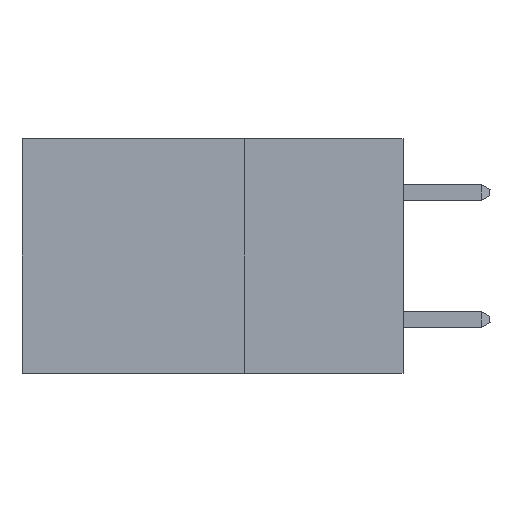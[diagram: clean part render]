
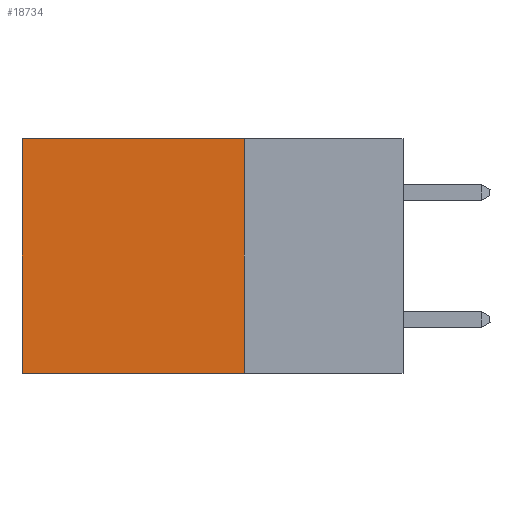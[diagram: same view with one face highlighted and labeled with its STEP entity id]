
A CAD part, left-side view. The second image highlights one B-rep face of the part: STEP entity #18734.
In plain terms, the highlighted planar face has unit normal (-1, 0, 0).
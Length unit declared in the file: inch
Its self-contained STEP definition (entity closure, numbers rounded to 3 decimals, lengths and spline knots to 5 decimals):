
#286 = LINE ( 'NONE', #6013, #18347 ) ;
#1853 = DIRECTION ( 'NONE',  ( 0., 1., 0. ) ) ;
#3866 = ORIENTED_EDGE ( 'NONE', *, *, #15349, .F. ) ;
#4247 = CARTESIAN_POINT ( 'NONE',  ( 0.2875, 0.6, 0. ) ) ;
#4672 = PLANE ( 'NONE',  #9237 ) ;
#4732 = DIRECTION ( 'NONE',  ( 0., 0., -1. ) ) ;
#5670 = LINE ( 'NONE', #18935, #10501 ) ;
#6013 = CARTESIAN_POINT ( 'NONE',  ( 0.2875, 0.25, 0. ) ) ;
#6296 = VERTEX_POINT ( 'NONE', #9944 ) ;
#7270 = ORIENTED_EDGE ( 'NONE', *, *, #11937, .F. ) ;
#7334 = EDGE_CURVE ( 'NONE', #19395, #7934, #16659, .T. ) ;
#7934 = VERTEX_POINT ( 'NONE', #17680 ) ;
#8270 = CARTESIAN_POINT ( 'NONE',  ( 0.2875, 0.25, 0. ) ) ;
#9197 = VECTOR ( 'NONE', #18101, 39.37008 ) ;
#9237 = AXIS2_PLACEMENT_3D ( 'NONE', #18799, #9454, #4732 ) ;
#9454 = DIRECTION ( 'NONE',  ( 1., 0., 0. ) ) ;
#9944 = CARTESIAN_POINT ( 'NONE',  ( 0.2875, 0.25, -0.37 ) ) ;
#9947 = DIRECTION ( 'NONE',  ( 0., 1., 0. ) ) ;
#9979 = VERTEX_POINT ( 'NONE', #16323 ) ;
#10481 = LINE ( 'NONE', #8270, #17430 ) ;
#10501 = VECTOR ( 'NONE', #1853, 39.37008 ) ;
#10537 = DIRECTION ( 'NONE',  ( 0., 0., -1. ) ) ;
#11758 = FACE_OUTER_BOUND ( 'NONE', #12238, .T. ) ;
#11937 = EDGE_CURVE ( 'NONE', #6296, #7934, #5670, .T. ) ;
#12238 = EDGE_LOOP ( 'NONE', ( #15682, #7270, #3866, #17017 ) ) ;
#12253 = EDGE_CURVE ( 'NONE', #9979, #19395, #10481, .T. ) ;
#15349 = EDGE_CURVE ( 'NONE', #9979, #6296, #286, .T. ) ;
#15682 = ORIENTED_EDGE ( 'NONE', *, *, #7334, .T. ) ;
#16323 = CARTESIAN_POINT ( 'NONE',  ( 0.2875, 0.25, 0. ) ) ;
#16659 = LINE ( 'NONE', #4247, #9197 ) ;
#17017 = ORIENTED_EDGE ( 'NONE', *, *, #12253, .T. ) ;
#17430 = VECTOR ( 'NONE', #9947, 39.37008 ) ;
#17680 = CARTESIAN_POINT ( 'NONE',  ( 0.2875, 0.6, -0.37 ) ) ;
#18101 = DIRECTION ( 'NONE',  ( 0., 0., -1. ) ) ;
#18347 = VECTOR ( 'NONE', #10537, 39.37008 ) ;
#18734 = ADVANCED_FACE ( 'NONE', ( #11758 ), #4672, .F. ) ;
#18799 = CARTESIAN_POINT ( 'NONE',  ( 0.2875, 0.25, 0. ) ) ;
#18935 = CARTESIAN_POINT ( 'NONE',  ( 0.2875, 0.25, -0.37 ) ) ;
#19163 = CARTESIAN_POINT ( 'NONE',  ( 0.2875, 0.6, 0. ) ) ;
#19395 = VERTEX_POINT ( 'NONE', #19163 ) ;
